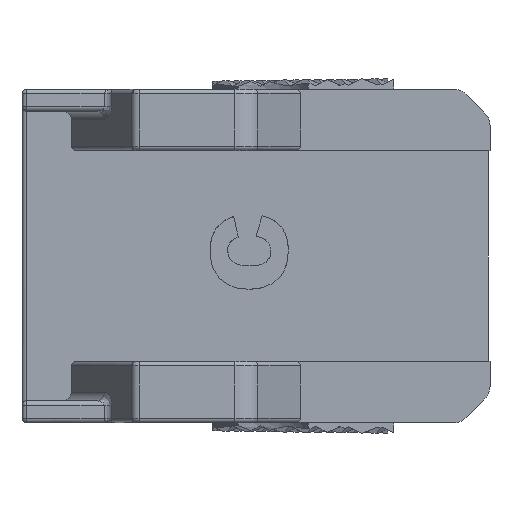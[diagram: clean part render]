
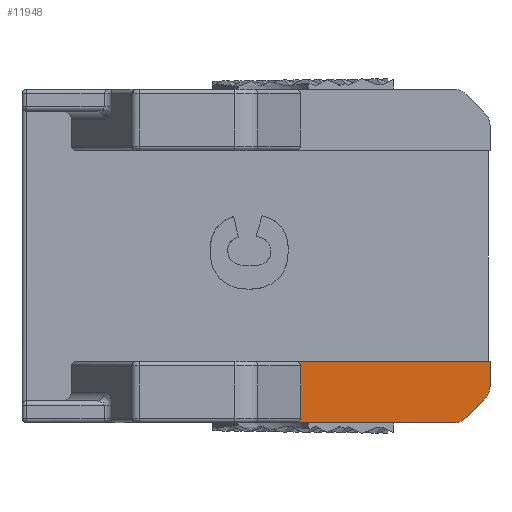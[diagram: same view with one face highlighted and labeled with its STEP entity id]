
A CAD part, left-side view. The second image highlights one B-rep face of the part: STEP entity #11948.
In plain terms, the highlighted planar face has unit normal (-1, 0, 0).
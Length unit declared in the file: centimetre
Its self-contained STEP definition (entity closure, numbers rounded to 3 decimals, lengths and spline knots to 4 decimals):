
#271=LINE($,#17480,#1641);
#296=LINE($,#17625,#1666);
#297=LINE($,#17629,#1667);
#298=LINE($,#17632,#1668);
#299=LINE($,#17633,#1669);
#1641=VECTOR($,#13767,0.287);
#1666=VECTOR($,#13846,2.2157);
#1667=VECTOR($,#13849,0.6);
#1668=VECTOR($,#13852,1.8011);
#1669=VECTOR($,#13853,0.3018);
#2968=PLANE($,#12749);
#3513=ELLIPSE($,#12742,0.2008,0.2);
#3514=ELLIPSE($,#12745,0.2008,0.2);
#3515=ELLIPSE($,#12750,0.0577,0.05);
#3516=ELLIPSE($,#12751,0.0577,0.05);
#3679=FACE_OUTER_BOUND($,#4449,.T.);
#4449=EDGE_LOOP($,(#8543,#8544,#8545,#8546,#8547,#8548,#8549,#8550,#8551));
#5594=VERTEX_POINT($,#17477);
#5595=VERTEX_POINT($,#17479);
#5628=VERTEX_POINT($,#17585);
#5630=VERTEX_POINT($,#17591);
#5631=VERTEX_POINT($,#17593);
#5632=VERTEX_POINT($,#17624);
#5633=VERTEX_POINT($,#17626);
#5634=VERTEX_POINT($,#17628);
#5635=VERTEX_POINT($,#17630);
#6648=EDGE_CURVE($,#5594,#5595,#271,.F.);
#6687=EDGE_CURVE($,#5595,#5628,#3513,.T.);
#6691=EDGE_CURVE($,#5630,#5631,#3514,.T.);
#6696=EDGE_CURVE($,#5594,#5632,#296,.T.);
#6697=EDGE_CURVE($,#5633,#5632,#3515,.T.);
#6698=EDGE_CURVE($,#5633,#5634,#297,.F.);
#6699=EDGE_CURVE($,#5634,#5635,#3516,.T.);
#6700=EDGE_CURVE($,#5631,#5635,#298,.T.);
#6701=EDGE_CURVE($,#5628,#5630,#299,.T.);
#8543=ORIENTED_EDGE($,*,*,#6687,.F.);
#8544=ORIENTED_EDGE($,*,*,#6648,.F.);
#8545=ORIENTED_EDGE($,*,*,#6696,.T.);
#8546=ORIENTED_EDGE($,*,*,#6697,.F.);
#8547=ORIENTED_EDGE($,*,*,#6698,.T.);
#8548=ORIENTED_EDGE($,*,*,#6699,.T.);
#8549=ORIENTED_EDGE($,*,*,#6700,.F.);
#8550=ORIENTED_EDGE($,*,*,#6691,.F.);
#8551=ORIENTED_EDGE($,*,*,#6701,.F.);
#11948=ADVANCED_FACE($,(#3679),#2968,.T.);
#12742=AXIS2_PLACEMENT_3D($,#17586,#13827,#13828);
#12745=AXIS2_PLACEMENT_3D($,#17594,#13835,#13836);
#12749=AXIS2_PLACEMENT_3D($,#17623,#13844,#13845);
#12750=AXIS2_PLACEMENT_3D($,#17627,#13847,#13848);
#12751=AXIS2_PLACEMENT_3D($,#17631,#13850,#13851);
#13767=DIRECTION($,(0.,0.,1.));
#13827=DIRECTION('center_axis',(1.,0.,0.));
#13828=DIRECTION('ref_axis',(0.,-1.,0.));
#13835=DIRECTION('center_axis',(1.,0.,0.));
#13836=DIRECTION('ref_axis',(0.,-1.,0.));
#13844=DIRECTION('center_axis',(-1.,0.,0.));
#13845=DIRECTION('ref_axis',(0.,1.,0.));
#13846=DIRECTION($,(0.,1.,0.));
#13847=DIRECTION('center_axis',(-1.,0.,0.));
#13848=DIRECTION('ref_axis',(0.,-1.,0.));
#13849=DIRECTION($,(0.,0.,1.));
#13850=DIRECTION('center_axis',(1.,0.,0.));
#13851=DIRECTION('ref_axis',(0.,-1.,0.));
#13852=DIRECTION($,(0.,1.,0.));
#13853=DIRECTION($,(0.,0.708,-0.706));
#17477=CARTESIAN_POINT('',(-8.48,-6.1222,-1.1));
#17479=CARTESIAN_POINT('',(-8.48,-6.1222,-1.387));
#17480=CARTESIAN_POINT($,(-8.48,-6.1222,0.9133));
#17585=CARTESIAN_POINT('',(-8.48,-6.0634,-1.5284));
#17586=CARTESIAN_POINT('Origin',(-8.48,-5.9215,-1.387));
#17591=CARTESIAN_POINT('',(-8.48,-5.8496,-1.7414));
#17593=CARTESIAN_POINT('',(-8.48,-5.7076,-1.8));
#17594=CARTESIAN_POINT('Origin',(-8.48,-5.7076,-1.6));
#17623=CARTESIAN_POINT('Origin',(-8.48,-4.2876,1.7266));
#17624=CARTESIAN_POINT('',(-8.48,-3.9066,-1.1));
#17625=CARTESIAN_POINT($,(-8.48,-3.7231,-1.1));
#17626=CARTESIAN_POINT('',(-8.48,-3.9643,-1.15));
#17627=CARTESIAN_POINT('Origin',(-8.48,-3.9066,-1.15));
#17628=CARTESIAN_POINT('',(-8.48,-3.9643,-1.75));
#17629=CARTESIAN_POINT($,(-8.48,-3.9643,-0.0967));
#17630=CARTESIAN_POINT('',(-8.48,-3.9066,-1.8));
#17631=CARTESIAN_POINT('Origin',(-8.48,-3.9066,-1.75));
#17632=CARTESIAN_POINT($,(-8.48,-3.8524,-1.8));
#17633=CARTESIAN_POINT($,(-8.48,-6.2154,-1.377));
